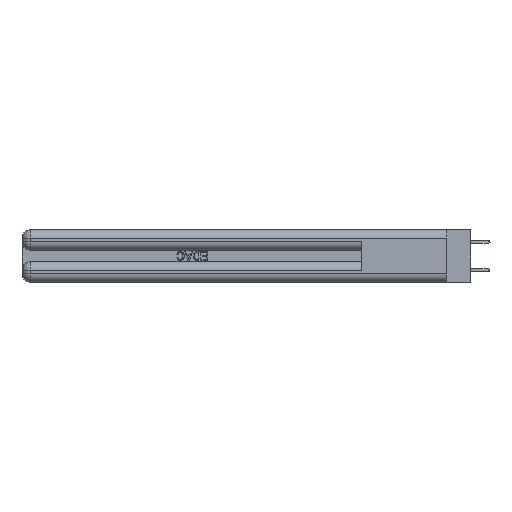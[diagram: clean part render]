
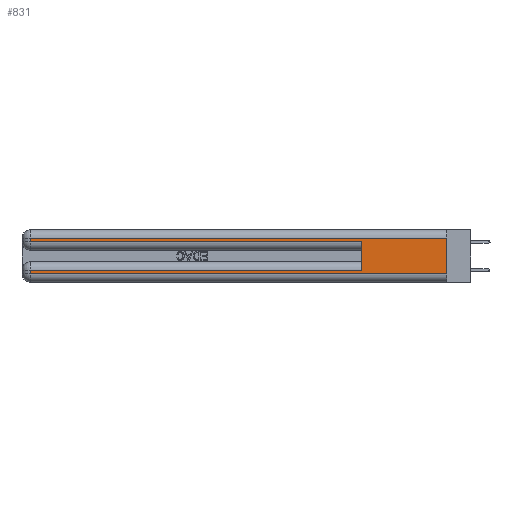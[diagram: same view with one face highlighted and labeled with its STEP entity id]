
A CAD part, left-side view. The second image highlights one B-rep face of the part: STEP entity #831.
In plain terms, the highlighted planar face has unit normal (-1, 0, 0).
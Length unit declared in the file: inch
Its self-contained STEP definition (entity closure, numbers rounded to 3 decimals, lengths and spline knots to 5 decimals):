
#271 = CARTESIAN_POINT ( 'NONE',  ( 0., 0., 0.37 ) ) ;
#831 = ADVANCED_FACE ( 'NONE', ( #14670 ), #25138, .F. ) ;
#914 = LINE ( 'NONE', #41370, #25922 ) ;
#1026 = CARTESIAN_POINT ( 'NONE',  ( 0., 2.94, 0.085 ) ) ;
#1307 = CARTESIAN_POINT ( 'NONE',  ( 0., 0.6, 0.145 ) ) ;
#1385 = CARTESIAN_POINT ( 'NONE',  ( 0., 0., 0.31 ) ) ;
#2266 = VECTOR ( 'NONE', #46363, 39.37008 ) ;
#3960 = DIRECTION ( 'NONE',  ( 1., 0., 0. ) ) ;
#6868 = CARTESIAN_POINT ( 'NONE',  ( 0., 2.94, 0.37 ) ) ;
#7309 = EDGE_CURVE ( 'NONE', #43634, #34212, #16652, .T. ) ;
#8640 = VERTEX_POINT ( 'NONE', #20318 ) ;
#8646 = EDGE_CURVE ( 'NONE', #27960, #8640, #39313, .T. ) ;
#10723 = CARTESIAN_POINT ( 'NONE',  ( 0., 0.6, 0.285 ) ) ;
#11633 = VECTOR ( 'NONE', #12268, 39.37008 ) ;
#12268 = DIRECTION ( 'NONE',  ( 0., 0., -1. ) ) ;
#13645 = AXIS2_PLACEMENT_3D ( 'NONE', #271, #3960, #18565 ) ;
#14670 = FACE_OUTER_BOUND ( 'NONE', #39303, .T. ) ;
#15318 = CARTESIAN_POINT ( 'NONE',  ( 0., 0., 0.31 ) ) ;
#15549 = LINE ( 'NONE', #15318, #18947 ) ;
#16075 = VERTEX_POINT ( 'NONE', #1026 ) ;
#16391 = VERTEX_POINT ( 'NONE', #26786 ) ;
#16446 = VERTEX_POINT ( 'NONE', #38005 ) ;
#16652 = LINE ( 'NONE', #1307, #2266 ) ;
#17421 = CARTESIAN_POINT ( 'NONE',  ( 0., 0., 0.085 ) ) ;
#18565 = DIRECTION ( 'NONE',  ( 0., 0., -1. ) ) ;
#18947 = VECTOR ( 'NONE', #37951, 39.37008 ) ;
#19198 = DIRECTION ( 'NONE',  ( 0., -1., 0. ) ) ;
#19464 = CARTESIAN_POINT ( 'NONE',  ( 0., 0., 0.06 ) ) ;
#19669 = LINE ( 'NONE', #17421, #27511 ) ;
#20318 = CARTESIAN_POINT ( 'NONE',  ( 0., 0., 0.06 ) ) ;
#21076 = DIRECTION ( 'NONE',  ( 0., 1., 0. ) ) ;
#22844 = EDGE_CURVE ( 'NONE', #45145, #16446, #45745, .T. ) ;
#24061 = EDGE_CURVE ( 'NONE', #16075, #16391, #40244, .T. ) ;
#24445 = ORIENTED_EDGE ( 'NONE', *, *, #8646, .F. ) ;
#24650 = EDGE_CURVE ( 'NONE', #43634, #16075, #19669, .T. ) ;
#25138 = PLANE ( 'NONE',  #13645 ) ;
#25922 = VECTOR ( 'NONE', #19198, 39.37008 ) ;
#26786 = CARTESIAN_POINT ( 'NONE',  ( 0., 2.94, 0.06 ) ) ;
#27009 = ORIENTED_EDGE ( 'NONE', *, *, #7309, .F. ) ;
#27511 = VECTOR ( 'NONE', #21076, 39.37008 ) ;
#27607 = CARTESIAN_POINT ( 'NONE',  ( 0., 0., 0.37 ) ) ;
#27960 = VERTEX_POINT ( 'NONE', #1385 ) ;
#28850 = ORIENTED_EDGE ( 'NONE', *, *, #24061, .T. ) ;
#29823 = CARTESIAN_POINT ( 'NONE',  ( 0., 2.94, 0.31 ) ) ;
#31446 = CARTESIAN_POINT ( 'NONE',  ( 0., 0.6, 0.085 ) ) ;
#34212 = VERTEX_POINT ( 'NONE', #10723 ) ;
#34567 = LINE ( 'NONE', #19464, #43393 ) ;
#36200 = ORIENTED_EDGE ( 'NONE', *, *, #37628, .T. ) ;
#36585 = DIRECTION ( 'NONE',  ( 0., 0., -1. ) ) ;
#37260 = CARTESIAN_POINT ( 'NONE',  ( 0., 2.94, 0.37 ) ) ;
#37628 = EDGE_CURVE ( 'NONE', #27960, #45145, #15549, .T. ) ;
#37641 = EDGE_CURVE ( 'NONE', #16446, #34212, #914, .T. ) ;
#37951 = DIRECTION ( 'NONE',  ( 0., 1., 0. ) ) ;
#37977 = DIRECTION ( 'NONE',  ( 0., -1., 0. ) ) ;
#38005 = CARTESIAN_POINT ( 'NONE',  ( 0., 2.94, 0.285 ) ) ;
#39303 = EDGE_LOOP ( 'NONE', ( #24445, #36200, #39444, #47326, #27009, #43483, #28850, #47615 ) ) ;
#39313 = LINE ( 'NONE', #27607, #11633 ) ;
#39444 = ORIENTED_EDGE ( 'NONE', *, *, #22844, .T. ) ;
#40244 = LINE ( 'NONE', #6868, #45309 ) ;
#41370 = CARTESIAN_POINT ( 'NONE',  ( 0., 0., 0.285 ) ) ;
#43393 = VECTOR ( 'NONE', #37977, 39.37008 ) ;
#43483 = ORIENTED_EDGE ( 'NONE', *, *, #24650, .T. ) ;
#43634 = VERTEX_POINT ( 'NONE', #31446 ) ;
#44335 = EDGE_CURVE ( 'NONE', #16391, #8640, #34567, .T. ) ;
#45145 = VERTEX_POINT ( 'NONE', #29823 ) ;
#45261 = DIRECTION ( 'NONE',  ( 0., 0., -1. ) ) ;
#45309 = VECTOR ( 'NONE', #36585, 39.37008 ) ;
#45745 = LINE ( 'NONE', #37260, #46051 ) ;
#46051 = VECTOR ( 'NONE', #45261, 39.37008 ) ;
#46363 = DIRECTION ( 'NONE',  ( 0., 0., 1. ) ) ;
#47326 = ORIENTED_EDGE ( 'NONE', *, *, #37641, .T. ) ;
#47615 = ORIENTED_EDGE ( 'NONE', *, *, #44335, .T. ) ;
